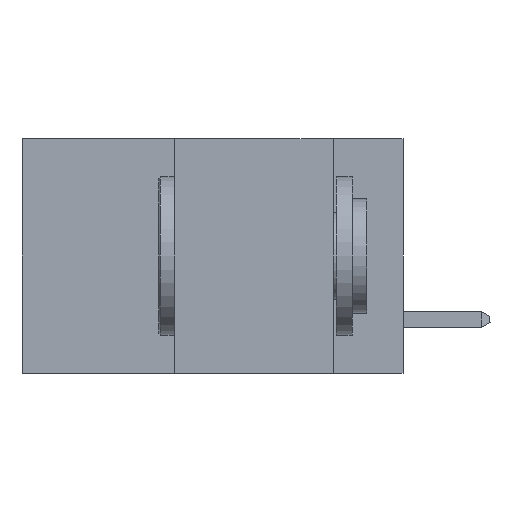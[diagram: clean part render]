
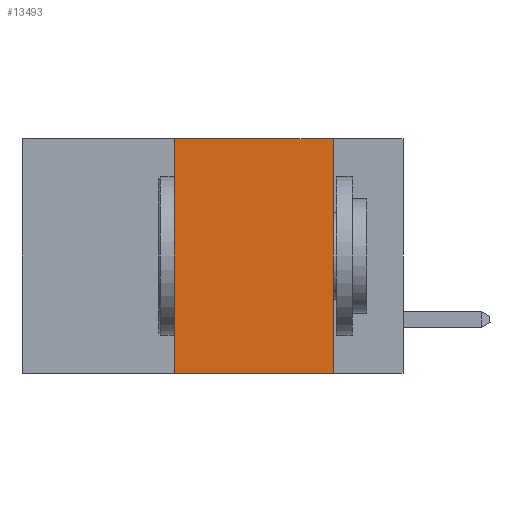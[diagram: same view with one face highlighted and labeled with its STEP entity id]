
A CAD part, left-side view. The second image highlights one B-rep face of the part: STEP entity #13493.
In plain terms, the highlighted planar face has unit normal (-1, 0, 0).
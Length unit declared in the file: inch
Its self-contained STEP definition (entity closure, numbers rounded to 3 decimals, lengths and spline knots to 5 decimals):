
#1805 = CARTESIAN_POINT ( 'NONE',  ( 0., 0.36, 0. ) ) ;
#1981 = VECTOR ( 'NONE', #8279, 39.37008 ) ;
#3907 = LINE ( 'NONE', #26565, #12069 ) ;
#5075 = LINE ( 'NONE', #43126, #21920 ) ;
#5350 = EDGE_CURVE ( 'NONE', #22882, #27836, #12482, .T. ) ;
#7364 = DIRECTION ( 'NONE',  ( 0., 0., -1. ) ) ;
#7663 = CARTESIAN_POINT ( 'NONE',  ( 0., 0.11, 0. ) ) ;
#8279 = DIRECTION ( 'NONE',  ( 0., 0., 1. ) ) ;
#9137 = CARTESIAN_POINT ( 'NONE',  ( 0., 0.36, -0.37 ) ) ;
#12069 = VECTOR ( 'NONE', #16129, 39.37008 ) ;
#12482 = LINE ( 'NONE', #41748, #37896 ) ;
#13493 = ADVANCED_FACE ( 'NONE', ( #13813 ), #16421, .F. ) ;
#13813 = FACE_OUTER_BOUND ( 'NONE', #40200, .T. ) ;
#13907 = VERTEX_POINT ( 'NONE', #23628 ) ;
#14068 = CARTESIAN_POINT ( 'NONE',  ( 0., 0.11, -0.37 ) ) ;
#14906 = LINE ( 'NONE', #1805, #1981 ) ;
#16129 = DIRECTION ( 'NONE',  ( 0., -1., 0. ) ) ;
#16421 = PLANE ( 'NONE',  #29825 ) ;
#17662 = EDGE_CURVE ( 'NONE', #42233, #27836, #3907, .T. ) ;
#19483 = DIRECTION ( 'NONE',  ( 0., 0., -1. ) ) ;
#21920 = VECTOR ( 'NONE', #36325, 39.37008 ) ;
#22882 = VERTEX_POINT ( 'NONE', #7663 ) ;
#23184 = ORIENTED_EDGE ( 'NONE', *, *, #17662, .T. ) ;
#23204 = DIRECTION ( 'NONE',  ( 1., 0., 0. ) ) ;
#23628 = CARTESIAN_POINT ( 'NONE',  ( 0., 0.36, 0. ) ) ;
#26565 = CARTESIAN_POINT ( 'NONE',  ( 0., 0.6, -0.37 ) ) ;
#27836 = VERTEX_POINT ( 'NONE', #14068 ) ;
#28012 = ORIENTED_EDGE ( 'NONE', *, *, #35850, .F. ) ;
#29825 = AXIS2_PLACEMENT_3D ( 'NONE', #33357, #23204, #19483 ) ;
#33357 = CARTESIAN_POINT ( 'NONE',  ( 0., 0.6, 0. ) ) ;
#34197 = ORIENTED_EDGE ( 'NONE', *, *, #5350, .F. ) ;
#35850 = EDGE_CURVE ( 'NONE', #42233, #13907, #14906, .T. ) ;
#36325 = DIRECTION ( 'NONE',  ( 0., -1., 0. ) ) ;
#37242 = EDGE_CURVE ( 'NONE', #13907, #22882, #5075, .T. ) ;
#37896 = VECTOR ( 'NONE', #7364, 39.37008 ) ;
#37913 = ORIENTED_EDGE ( 'NONE', *, *, #37242, .F. ) ;
#40200 = EDGE_LOOP ( 'NONE', ( #34197, #37913, #28012, #23184 ) ) ;
#41748 = CARTESIAN_POINT ( 'NONE',  ( 0., 0.11, 0. ) ) ;
#42233 = VERTEX_POINT ( 'NONE', #9137 ) ;
#43126 = CARTESIAN_POINT ( 'NONE',  ( 0., 0.6, 0. ) ) ;
